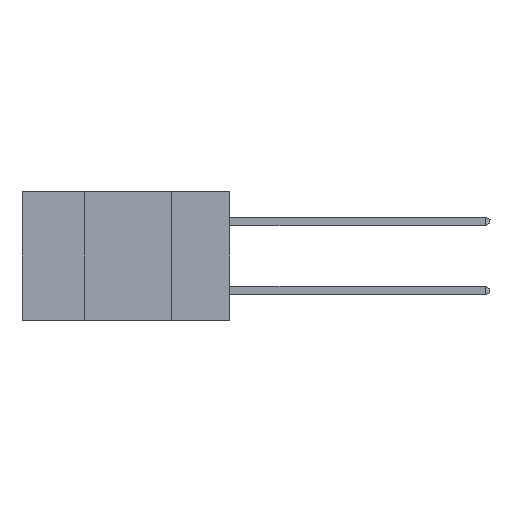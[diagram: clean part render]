
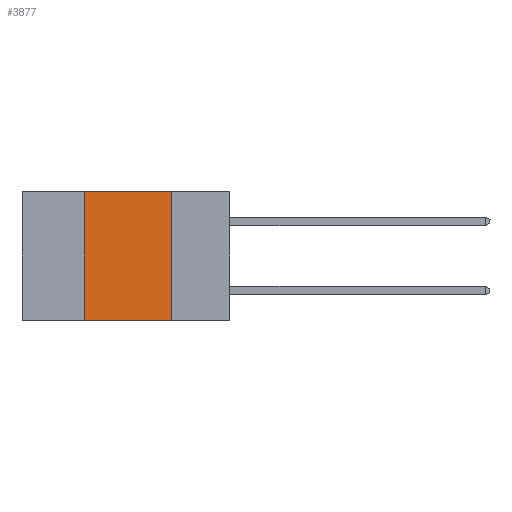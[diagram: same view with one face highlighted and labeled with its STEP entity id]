
A CAD part, left-side view. The second image highlights one B-rep face of the part: STEP entity #3877.
In plain terms, the highlighted planar face has unit normal (-1, 0, 0).
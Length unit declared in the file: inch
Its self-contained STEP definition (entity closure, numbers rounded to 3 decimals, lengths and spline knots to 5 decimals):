
#58 = DIRECTION ( 'NONE',  ( 0., -1., 0. ) ) ;
#166 = ORIENTED_EDGE ( 'NONE', *, *, #14583, .T. ) ;
#349 = VECTOR ( 'NONE', #2159, 39.37008 ) ;
#1130 = CARTESIAN_POINT ( 'NONE',  ( 0., 0.17, 0. ) ) ;
#1945 = ORIENTED_EDGE ( 'NONE', *, *, #11920, .F. ) ;
#2159 = DIRECTION ( 'NONE',  ( 0., -1., 0. ) ) ;
#2185 = VECTOR ( 'NONE', #15848, 39.37008 ) ;
#2346 = VERTEX_POINT ( 'NONE', #17420 ) ;
#3633 = EDGE_LOOP ( 'NONE', ( #9652, #13582, #1945, #166 ) ) ;
#3877 = ADVANCED_FACE ( 'NONE', ( #16195 ), #25313, .F. ) ;
#3908 = CARTESIAN_POINT ( 'NONE',  ( 0., 0.17, -0.37 ) ) ;
#4128 = VERTEX_POINT ( 'NONE', #9860 ) ;
#7261 = AXIS2_PLACEMENT_3D ( 'NONE', #17271, #20886, #16991 ) ;
#7635 = EDGE_CURVE ( 'NONE', #8789, #14634, #13841, .T. ) ;
#7881 = DIRECTION ( 'NONE',  ( 0., 0., 1. ) ) ;
#8435 = VECTOR ( 'NONE', #7881, 39.37008 ) ;
#8460 = VECTOR ( 'NONE', #58, 39.37008 ) ;
#8789 = VERTEX_POINT ( 'NONE', #1130 ) ;
#9652 = ORIENTED_EDGE ( 'NONE', *, *, #7635, .F. ) ;
#9860 = CARTESIAN_POINT ( 'NONE',  ( 0., 0.42, 0. ) ) ;
#10193 = CARTESIAN_POINT ( 'NONE',  ( 0., 0.17, -0.37 ) ) ;
#11003 = EDGE_CURVE ( 'NONE', #4128, #8789, #22184, .T. ) ;
#11920 = EDGE_CURVE ( 'NONE', #2346, #4128, #20360, .T. ) ;
#13582 = ORIENTED_EDGE ( 'NONE', *, *, #11003, .F. ) ;
#13841 = LINE ( 'NONE', #3908, #2185 ) ;
#14583 = EDGE_CURVE ( 'NONE', #2346, #14634, #21374, .T. ) ;
#14634 = VERTEX_POINT ( 'NONE', #10193 ) ;
#15848 = DIRECTION ( 'NONE',  ( 0., 0., -1. ) ) ;
#15938 = CARTESIAN_POINT ( 'NONE',  ( 0., 0.42, -0.37 ) ) ;
#16195 = FACE_OUTER_BOUND ( 'NONE', #3633, .T. ) ;
#16991 = DIRECTION ( 'NONE',  ( 0., 0., -1. ) ) ;
#17271 = CARTESIAN_POINT ( 'NONE',  ( 0., 0.6, 0. ) ) ;
#17420 = CARTESIAN_POINT ( 'NONE',  ( 0., 0.42, -0.37 ) ) ;
#18023 = CARTESIAN_POINT ( 'NONE',  ( 0., 0.6, 0. ) ) ;
#19227 = CARTESIAN_POINT ( 'NONE',  ( 0., 0.6, -0.37 ) ) ;
#20360 = LINE ( 'NONE', #15938, #8435 ) ;
#20886 = DIRECTION ( 'NONE',  ( 1., 0., 0. ) ) ;
#21374 = LINE ( 'NONE', #19227, #349 ) ;
#22184 = LINE ( 'NONE', #18023, #8460 ) ;
#25313 = PLANE ( 'NONE',  #7261 ) ;
